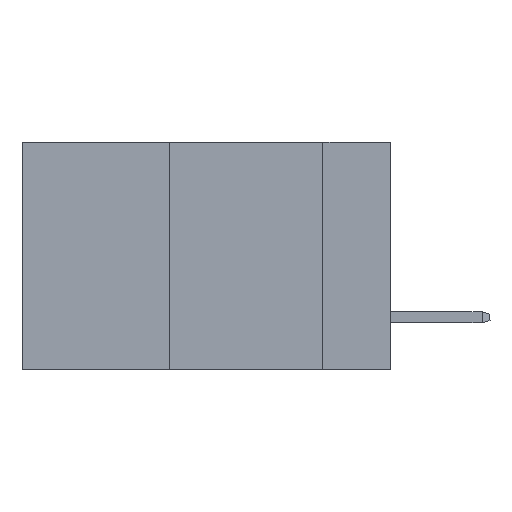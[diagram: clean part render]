
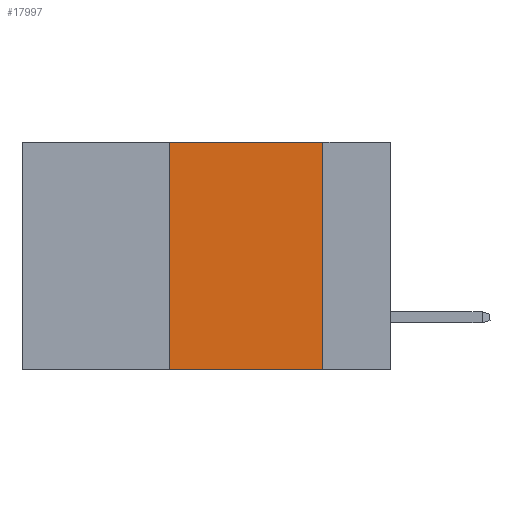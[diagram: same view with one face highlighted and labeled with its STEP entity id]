
A CAD part, left-side view. The second image highlights one B-rep face of the part: STEP entity #17997.
In plain terms, the highlighted planar face has unit normal (-1, 0, 0).
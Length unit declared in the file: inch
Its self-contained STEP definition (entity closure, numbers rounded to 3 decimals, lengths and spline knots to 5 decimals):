
#602 = EDGE_CURVE ( 'NONE', #12206, #16945, #685, .T. ) ;
#685 = LINE ( 'NONE', #5267, #6531 ) ;
#993 = CARTESIAN_POINT ( 'NONE',  ( 0., 0.11, -0.37 ) ) ;
#2018 = ORIENTED_EDGE ( 'NONE', *, *, #18579, .T. ) ;
#2876 = DIRECTION ( 'NONE',  ( 0., 0., 1. ) ) ;
#3163 = CARTESIAN_POINT ( 'NONE',  ( 0., 0.6, -0.37 ) ) ;
#3355 = PLANE ( 'NONE',  #10433 ) ;
#3432 = CARTESIAN_POINT ( 'NONE',  ( 0., 0.6, 0. ) ) ;
#4494 = CARTESIAN_POINT ( 'NONE',  ( 0., 0.11, 0. ) ) ;
#4663 = CARTESIAN_POINT ( 'NONE',  ( 0., 0.36, 0. ) ) ;
#5210 = DIRECTION ( 'NONE',  ( 0., 0., -1. ) ) ;
#5267 = CARTESIAN_POINT ( 'NONE',  ( 0., 0.11, 0. ) ) ;
#5594 = DIRECTION ( 'NONE',  ( 0., 0., -1. ) ) ;
#6207 = DIRECTION ( 'NONE',  ( 0., -1., 0. ) ) ;
#6531 = VECTOR ( 'NONE', #5594, 39.37008 ) ;
#7244 = VECTOR ( 'NONE', #17075, 39.37008 ) ;
#9124 = CARTESIAN_POINT ( 'NONE',  ( 0., 0.36, 0. ) ) ;
#9735 = ORIENTED_EDGE ( 'NONE', *, *, #19643, .F. ) ;
#10433 = AXIS2_PLACEMENT_3D ( 'NONE', #3432, #15602, #5210 ) ;
#11551 = LINE ( 'NONE', #4663, #15012 ) ;
#11879 = LINE ( 'NONE', #3163, #7244 ) ;
#12206 = VERTEX_POINT ( 'NONE', #4494 ) ;
#14839 = ORIENTED_EDGE ( 'NONE', *, *, #19714, .F. ) ;
#15012 = VECTOR ( 'NONE', #2876, 39.37008 ) ;
#15101 = FACE_OUTER_BOUND ( 'NONE', #17506, .T. ) ;
#15397 = VERTEX_POINT ( 'NONE', #9124 ) ;
#15602 = DIRECTION ( 'NONE',  ( 1., 0., 0. ) ) ;
#16727 = VERTEX_POINT ( 'NONE', #21104 ) ;
#16945 = VERTEX_POINT ( 'NONE', #993 ) ;
#17075 = DIRECTION ( 'NONE',  ( 0., -1., 0. ) ) ;
#17506 = EDGE_LOOP ( 'NONE', ( #22295, #9735, #14839, #2018 ) ) ;
#17997 = ADVANCED_FACE ( 'NONE', ( #15101 ), #3355, .F. ) ;
#18579 = EDGE_CURVE ( 'NONE', #16727, #16945, #11879, .T. ) ;
#19643 = EDGE_CURVE ( 'NONE', #15397, #12206, #21678, .T. ) ;
#19714 = EDGE_CURVE ( 'NONE', #16727, #15397, #11551, .T. ) ;
#19992 = CARTESIAN_POINT ( 'NONE',  ( 0., 0.6, 0. ) ) ;
#21104 = CARTESIAN_POINT ( 'NONE',  ( 0., 0.36, -0.37 ) ) ;
#21152 = VECTOR ( 'NONE', #6207, 39.37008 ) ;
#21678 = LINE ( 'NONE', #19992, #21152 ) ;
#22295 = ORIENTED_EDGE ( 'NONE', *, *, #602, .F. ) ;
